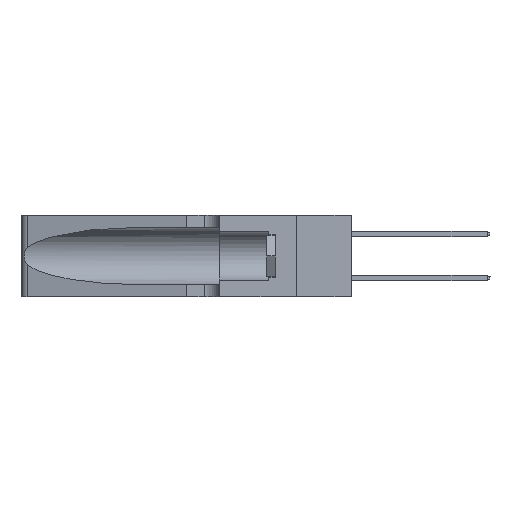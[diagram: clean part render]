
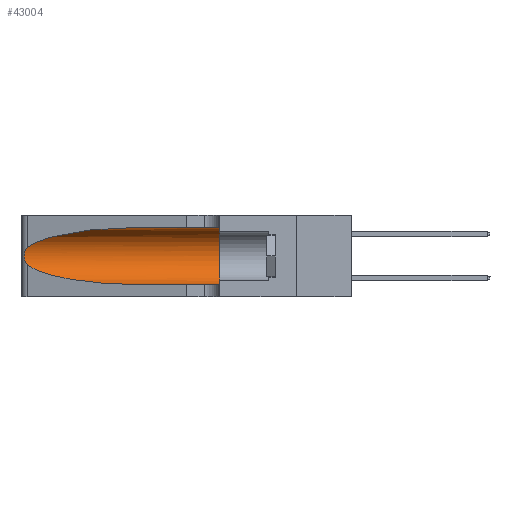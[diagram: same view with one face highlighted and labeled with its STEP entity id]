
A CAD part, left-side view. The second image highlights one B-rep face of the part: STEP entity #43004.
In plain terms, the highlighted cylindrical face has radius 3.308 mm (diameter 6.617 mm), a partial arc.
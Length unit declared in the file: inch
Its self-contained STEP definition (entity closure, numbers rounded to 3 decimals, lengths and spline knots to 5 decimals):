
#1064 = CARTESIAN_POINT ( 'NONE',  ( 0.1305, 0.35, 0.185 ) ) ;
#1430 = CARTESIAN_POINT ( 'NONE',  ( 0.1305, 0.72297, 0.31525 ) ) ;
#2421 = CARTESIAN_POINT ( 'NONE',  ( 0.25555, 1.22994, 0.2215 ) ) ;
#2566 = CARTESIAN_POINT ( 'NONE',  ( 0.25854, 1.2359, 0.20912 ) ) ;
#2622 = LINE ( 'NONE', #44136, #29619 ) ;
#4654 = DIRECTION ( 'NONE',  ( 0., 0., 1. ) ) ;
#5543 = EDGE_CURVE ( 'NONE', #19053, #41674, #21898, .T. ) ;
#5991 = ORIENTED_EDGE ( 'NONE', *, *, #37845, .F. ) ;
#6132 = CARTESIAN_POINT ( 'NONE',  ( 0.26075, 1.23896, 0.19203 ) ) ;
#6670 = CARTESIAN_POINT ( 'NONE',  ( 0.1305, 1.61858, 0.05475 ) ) ;
#6812 = VECTOR ( 'NONE', #10291, 39.37008 ) ;
#7258 = ORIENTED_EDGE ( 'NONE', *, *, #5543, .T. ) ;
#8621 = CARTESIAN_POINT ( 'NONE',  ( 0.25487, 1.22718, 0.22369 ) ) ;
#9713 = CARTESIAN_POINT ( 'NONE',  ( 0.2373, 1.15595, 0.08982 ) ) ;
#9733 = CARTESIAN_POINT ( 'NONE',  ( 0.26017, 1.23833, 0.17102 ) ) ;
#10291 = DIRECTION ( 'NONE',  ( 0., -1., 0. ) ) ;
#13293 = CARTESIAN_POINT ( 'NONE',  ( 0.1305, 0.72297, 0.05475 ) ) ;
#13319 = CARTESIAN_POINT ( 'NONE',  ( 0.25789, 1.23486, 0.15765 ) ) ;
#13659 = DIRECTION ( 'NONE',  ( 0., 0., -1. ) ) ;
#14087 = CARTESIAN_POINT ( 'NONE',  ( 0.1305, 0.72297, 0.05475 ) ) ;
#15445 = CARTESIAN_POINT ( 'NONE',  ( 0.1305, 0.35, 0.31525 ) ) ;
#16036 = CARTESIAN_POINT ( 'NONE',  ( 0.1305, 0.35, 0.05475 ) ) ;
#16283 = LINE ( 'NONE', #6670, #6812 ) ;
#16788 = VERTEX_POINT ( 'NONE', #16036 ) ;
#16871 = CARTESIAN_POINT ( 'NONE',  ( 0.25555, 1.22993, 0.14849 ) ) ;
#17327 = VERTEX_POINT ( 'NONE', #29091 ) ;
#17369 = EDGE_LOOP ( 'NONE', ( #17825, #33324, #7258, #28000, #24807, #5991 ) ) ;
#17725 = CYLINDRICAL_SURFACE ( 'NONE', #30815, 0.13025 ) ;
#17825 = ORIENTED_EDGE ( 'NONE', *, *, #35517, .T. ) ;
#18535 = B_SPLINE_CURVE_WITH_KNOTS ( 'NONE', 3,
 ( #37611, #2421, #44665, #23739, #2566, #27238, #6132, #30772, #9733, #34264, #13319, #37756, #16871, #41263 ),
 .UNSPECIFIED., .F., .F.,
 ( 4, 2, 2, 2, 2, 2, 4 ),
 ( 0., 0.00027, 0.00053, 0.00107, 0.0016, 0.00187, 0.00214 ),
 .UNSPECIFIED. ) ;
#18895 = EDGE_CURVE ( 'NONE', #44258, #16788, #43358, .T. ) ;
#19053 = VERTEX_POINT ( 'NONE', #19542 ) ;
#19542 = CARTESIAN_POINT ( 'NONE',  ( 0.25487, 1.22718, 0.14631 ) ) ;
#19724 = DIRECTION ( 'NONE',  ( 0., -1., 0. ) ) ;
#20733 = DIRECTION ( 'NONE',  ( 0., -1., 0. ) ) ;
#21125 = CARTESIAN_POINT ( 'NONE',  ( 0.25487, 1.22718, 0.22369 ) ) ;
#21898 =( BOUNDED_CURVE ( )  B_SPLINE_CURVE ( 3, ( #44641, #9713, #34240, #13293 ),
 .UNSPECIFIED., .F., .T. ) 
 B_SPLINE_CURVE_WITH_KNOTS ( ( 4, 4 ),
 ( 3.44316, 4.71239 ),
 .UNSPECIFIED. ) 
 CURVE ( )  GEOMETRIC_REPRESENTATION_ITEM ( )  RATIONAL_B_SPLINE_CURVE ( ( 1., 0.87, 0.87, 1. ) ) 
 REPRESENTATION_ITEM ( '' )  );
#22624 = CARTESIAN_POINT ( 'NONE',  ( 0.18966, 0.96281, 0.31525 ) ) ;
#23739 = CARTESIAN_POINT ( 'NONE',  ( 0.25787, 1.23484, 0.2124 ) ) ;
#24245 = EDGE_CURVE ( 'NONE', #24426, #19053, #18535, .T. ) ;
#24426 = VERTEX_POINT ( 'NONE', #21125 ) ;
#24703 = FACE_OUTER_BOUND ( 'NONE', #17369, .T. ) ;
#24807 = ORIENTED_EDGE ( 'NONE', *, *, #18895, .F. ) ;
#25785 = DIRECTION ( 'NONE',  ( 0., 1., 0. ) ) ;
#27238 = CARTESIAN_POINT ( 'NONE',  ( 0.26018, 1.23835, 0.19895 ) ) ;
#28000 = ORIENTED_EDGE ( 'NONE', *, *, #40386, .T. ) ;
#29091 = CARTESIAN_POINT ( 'NONE',  ( 0.1305, 0.72297, 0.31525 ) ) ;
#29619 = VECTOR ( 'NONE', #19724, 39.37008 ) ;
#29625 = CARTESIAN_POINT ( 'NONE',  ( 0.2373, 1.15595, 0.28018 ) ) ;
#30772 = CARTESIAN_POINT ( 'NONE',  ( 0.26075, 1.23896, 0.178 ) ) ;
#30815 = AXIS2_PLACEMENT_3D ( 'NONE', #45147, #20733, #13659 ) ;
#31409 =( BOUNDED_CURVE ( )  B_SPLINE_CURVE ( 3, ( #1430, #22624, #29625, #8621 ),
 .UNSPECIFIED., .F., .F. ) 
 B_SPLINE_CURVE_WITH_KNOTS ( ( 4, 4 ),
 ( 1.5708, 2.84003 ),
 .UNSPECIFIED. ) 
 CURVE ( )  GEOMETRIC_REPRESENTATION_ITEM ( )  RATIONAL_B_SPLINE_CURVE ( ( 1., 0.87, 0.87, 1. ) ) 
 REPRESENTATION_ITEM ( '' )  );
#33324 = ORIENTED_EDGE ( 'NONE', *, *, #24245, .T. ) ;
#34240 = CARTESIAN_POINT ( 'NONE',  ( 0.18966, 0.96281, 0.05475 ) ) ;
#34264 = CARTESIAN_POINT ( 'NONE',  ( 0.25856, 1.23593, 0.16098 ) ) ;
#35517 = EDGE_CURVE ( 'NONE', #17327, #24426, #31409, .T. ) ;
#37611 = CARTESIAN_POINT ( 'NONE',  ( 0.25487, 1.22718, 0.22369 ) ) ;
#37756 = CARTESIAN_POINT ( 'NONE',  ( 0.25639, 1.23186, 0.15144 ) ) ;
#37845 = EDGE_CURVE ( 'NONE', #17327, #44258, #2622, .T. ) ;
#39883 = AXIS2_PLACEMENT_3D ( 'NONE', #1064, #25785, #4654 ) ;
#40386 = EDGE_CURVE ( 'NONE', #41674, #16788, #16283, .T. ) ;
#41263 = CARTESIAN_POINT ( 'NONE',  ( 0.25487, 1.22718, 0.14631 ) ) ;
#41674 = VERTEX_POINT ( 'NONE', #14087 ) ;
#43004 = ADVANCED_FACE ( 'NONE', ( #24703 ), #17725, .F. ) ;
#43358 = CIRCLE ( 'NONE', #39883, 0.13025 ) ;
#44136 = CARTESIAN_POINT ( 'NONE',  ( 0.1305, 1.61858, 0.31525 ) ) ;
#44258 = VERTEX_POINT ( 'NONE', #15445 ) ;
#44641 = CARTESIAN_POINT ( 'NONE',  ( 0.25487, 1.22718, 0.14631 ) ) ;
#44665 = CARTESIAN_POINT ( 'NONE',  ( 0.25639, 1.23184, 0.21858 ) ) ;
#45147 = CARTESIAN_POINT ( 'NONE',  ( 0.1305, 1.61858, 0.185 ) ) ;
